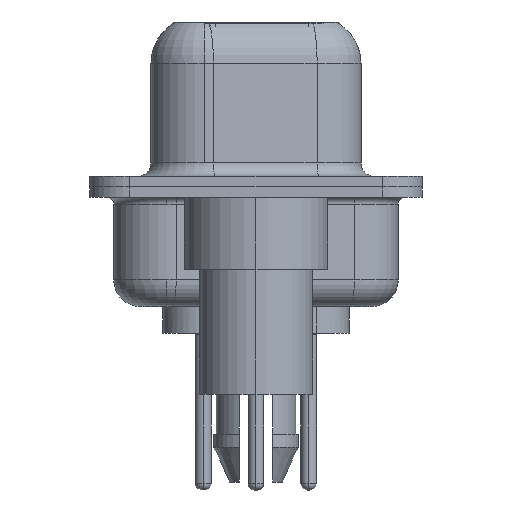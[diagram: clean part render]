
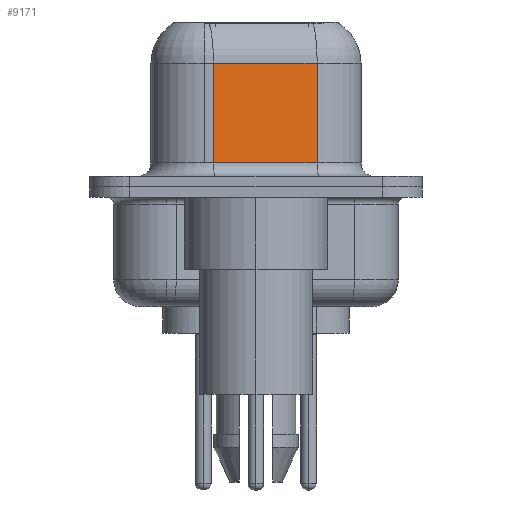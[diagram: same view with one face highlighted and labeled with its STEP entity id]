
A CAD part, left-side view. The second image highlights one B-rep face of the part: STEP entity #9171.
In plain terms, the highlighted planar face has unit normal (-0.985, -0.174, 0).
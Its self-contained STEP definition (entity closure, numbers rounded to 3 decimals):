
#255 = LINE ( 'NONE', #2366, #23070 ) ;
#978 = CARTESIAN_POINT ( 'NONE',  ( 4.38, 1.603, 0.9 ) ) ;
#1324 = ORIENTED_EDGE ( 'NONE', *, *, #21052, .T. ) ;
#1618 = CARTESIAN_POINT ( 'NONE',  ( 5.068, -2.297, 0.9 ) ) ;
#2366 = CARTESIAN_POINT ( 'NONE',  ( 4.38, 1.603, 6.4 ) ) ;
#2369 = ORIENTED_EDGE ( 'NONE', *, *, #15139, .T. ) ;
#2416 = EDGE_CURVE ( 'NONE', #15383, #20111, #21570, .T. ) ;
#3008 = VERTEX_POINT ( 'NONE', #21902 ) ;
#3300 = CARTESIAN_POINT ( 'NONE',  ( 5.068, -2.297, 4.65 ) ) ;
#3665 = CARTESIAN_POINT ( 'NONE',  ( 5.068, -2.297, 4.65 ) ) ;
#4817 = ORIENTED_EDGE ( 'NONE', *, *, #2416, .F. ) ;
#5491 = VECTOR ( 'NONE', #23697, 1000. ) ;
#5678 = EDGE_CURVE ( 'NONE', #9003, #20111, #10881, .T. ) ;
#5712 = VECTOR ( 'NONE', #16568, 1000. ) ;
#6076 = VECTOR ( 'NONE', #23451, 1000. ) ;
#7013 = PLANE ( 'NONE',  #12189 ) ;
#7980 = CARTESIAN_POINT ( 'NONE',  ( 5.068, -2.297, 0.9 ) ) ;
#8054 = EDGE_LOOP ( 'NONE', ( #4817, #2369, #1324, #9040 ) ) ;
#9003 = VERTEX_POINT ( 'NONE', #978 ) ;
#9040 = ORIENTED_EDGE ( 'NONE', *, *, #5678, .T. ) ;
#9171 = ADVANCED_FACE ( 'NONE', ( #14943 ), #7013, .F. ) ;
#10881 = LINE ( 'NONE', #1618, #5712 ) ;
#12189 = AXIS2_PLACEMENT_3D ( 'NONE', #24322, #18266, #18390 ) ;
#14943 = FACE_OUTER_BOUND ( 'NONE', #8054, .T. ) ;
#15139 = EDGE_CURVE ( 'NONE', #15383, #3008, #20225, .T. ) ;
#15383 = VERTEX_POINT ( 'NONE', #3665 ) ;
#16568 = DIRECTION ( 'NONE',  ( 0.174, -0.985, 0. ) ) ;
#17193 = DIRECTION ( 'NONE',  ( 0., 0., -1. ) ) ;
#18266 = DIRECTION ( 'NONE',  ( 0.985, 0.174, 0. ) ) ;
#18390 = DIRECTION ( 'NONE',  ( -0.174, 0.985, 0. ) ) ;
#20111 = VERTEX_POINT ( 'NONE', #7980 ) ;
#20225 = LINE ( 'NONE', #3300, #5491 ) ;
#21052 = EDGE_CURVE ( 'NONE', #3008, #9003, #255, .T. ) ;
#21570 = LINE ( 'NONE', #23206, #6076 ) ;
#21902 = CARTESIAN_POINT ( 'NONE',  ( 4.38, 1.603, 4.65 ) ) ;
#23070 = VECTOR ( 'NONE', #17193, 1000. ) ;
#23206 = CARTESIAN_POINT ( 'NONE',  ( 5.068, -2.297, 6.4 ) ) ;
#23451 = DIRECTION ( 'NONE',  ( 0., 0., -1. ) ) ;
#23697 = DIRECTION ( 'NONE',  ( -0.174, 0.985, 0. ) ) ;
#24322 = CARTESIAN_POINT ( 'NONE',  ( 5.068, -2.297, 6.4 ) ) ;
